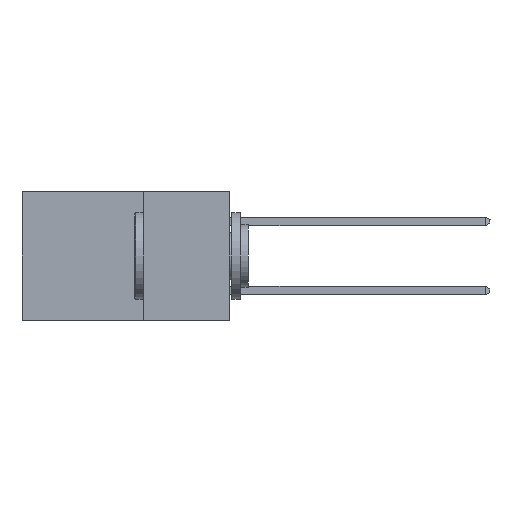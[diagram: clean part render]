
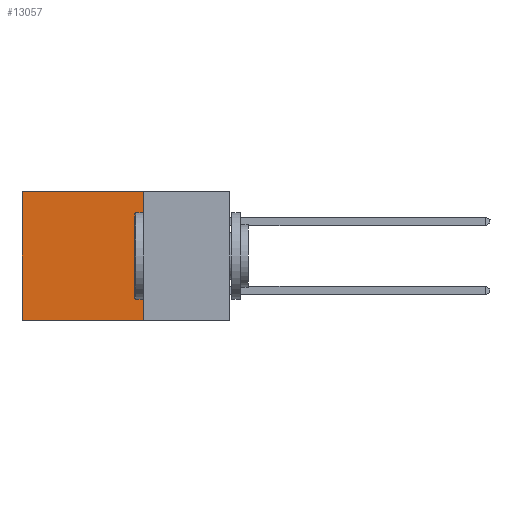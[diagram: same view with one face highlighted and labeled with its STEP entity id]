
A CAD part, left-side view. The second image highlights one B-rep face of the part: STEP entity #13057.
In plain terms, the highlighted planar face has unit normal (-1, 0, 0).
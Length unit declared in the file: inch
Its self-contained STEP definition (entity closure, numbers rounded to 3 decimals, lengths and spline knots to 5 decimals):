
#535 = CARTESIAN_POINT ( 'NONE',  ( 0.298, 0.25, 0. ) ) ;
#608 = CARTESIAN_POINT ( 'NONE',  ( 0.298, 0.25, 0. ) ) ;
#2200 = AXIS2_PLACEMENT_3D ( 'NONE', #608, #12230, #2263 ) ;
#2211 = ORIENTED_EDGE ( 'NONE', *, *, #14379, .F. ) ;
#2219 = CARTESIAN_POINT ( 'NONE',  ( 0.298, 0.6, 0. ) ) ;
#2263 = DIRECTION ( 'NONE',  ( 0., 0., -1. ) ) ;
#3460 = LINE ( 'NONE', #18662, #11784 ) ;
#3526 = FACE_OUTER_BOUND ( 'NONE', #17922, .T. ) ;
#3703 = ORIENTED_EDGE ( 'NONE', *, *, #4637, .T. ) ;
#3894 = ORIENTED_EDGE ( 'NONE', *, *, #13122, .T. ) ;
#4114 = DIRECTION ( 'NONE',  ( 0., 1., 0. ) ) ;
#4637 = EDGE_CURVE ( 'NONE', #14024, #7792, #15292, .T. ) ;
#5506 = DIRECTION ( 'NONE',  ( 0., 1., 0. ) ) ;
#6237 = CARTESIAN_POINT ( 'NONE',  ( 0.298, 0.6, 0. ) ) ;
#6260 = CARTESIAN_POINT ( 'NONE',  ( 0.298, 0.6, -0.37 ) ) ;
#6862 = DIRECTION ( 'NONE',  ( 0., 0., -1. ) ) ;
#7792 = VERTEX_POINT ( 'NONE', #6260 ) ;
#8483 = VECTOR ( 'NONE', #13759, 39.37008 ) ;
#8905 = ORIENTED_EDGE ( 'NONE', *, *, #13035, .F. ) ;
#9030 = CARTESIAN_POINT ( 'NONE',  ( 0.298, 0.25, -0.37 ) ) ;
#10234 = VERTEX_POINT ( 'NONE', #9030 ) ;
#10374 = VECTOR ( 'NONE', #6862, 39.37008 ) ;
#10411 = CARTESIAN_POINT ( 'NONE',  ( 0.298, 0.25, 0. ) ) ;
#10576 = PLANE ( 'NONE',  #2200 ) ;
#10713 = CARTESIAN_POINT ( 'NONE',  ( 0.298, 0.25, 0. ) ) ;
#11784 = VECTOR ( 'NONE', #5506, 39.37008 ) ;
#12230 = DIRECTION ( 'NONE',  ( 1., 0., 0. ) ) ;
#13035 = EDGE_CURVE ( 'NONE', #15071, #10234, #21096, .T. ) ;
#13057 = ADVANCED_FACE ( 'NONE', ( #3526 ), #10576, .F. ) ;
#13122 = EDGE_CURVE ( 'NONE', #15071, #14024, #15198, .T. ) ;
#13759 = DIRECTION ( 'NONE',  ( 0., 0., -1. ) ) ;
#14024 = VERTEX_POINT ( 'NONE', #6237 ) ;
#14379 = EDGE_CURVE ( 'NONE', #10234, #7792, #3460, .T. ) ;
#15071 = VERTEX_POINT ( 'NONE', #10411 ) ;
#15198 = LINE ( 'NONE', #10713, #19564 ) ;
#15292 = LINE ( 'NONE', #2219, #10374 ) ;
#17922 = EDGE_LOOP ( 'NONE', ( #3703, #2211, #8905, #3894 ) ) ;
#18662 = CARTESIAN_POINT ( 'NONE',  ( 0.298, 0.25, -0.37 ) ) ;
#19564 = VECTOR ( 'NONE', #4114, 39.37008 ) ;
#21096 = LINE ( 'NONE', #535, #8483 ) ;
